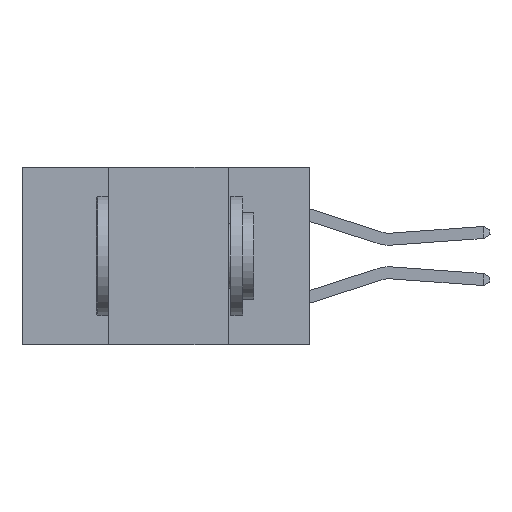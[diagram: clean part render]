
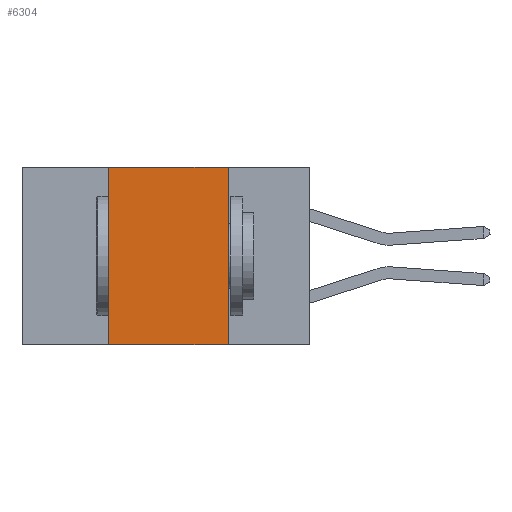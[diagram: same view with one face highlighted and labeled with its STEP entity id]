
A CAD part, left-side view. The second image highlights one B-rep face of the part: STEP entity #6304.
In plain terms, the highlighted planar face has unit normal (-1, 0, 0).
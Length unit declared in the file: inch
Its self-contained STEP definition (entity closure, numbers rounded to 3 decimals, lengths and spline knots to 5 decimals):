
#212 = DIRECTION ( 'NONE',  ( 0., 0., 1. ) ) ;
#338 = ORIENTED_EDGE ( 'NONE', *, *, #6580, .F. ) ;
#1374 = VERTEX_POINT ( 'NONE', #10463 ) ;
#1712 = LINE ( 'NONE', #11741, #5509 ) ;
#1825 = VECTOR ( 'NONE', #12276, 39.37008 ) ;
#3275 = VECTOR ( 'NONE', #7470, 39.37008 ) ;
#4083 = EDGE_CURVE ( 'NONE', #11158, #1374, #1712, .T. ) ;
#4914 = EDGE_CURVE ( 'NONE', #11158, #8663, #6254, .T. ) ;
#5231 = CARTESIAN_POINT ( 'NONE',  ( 0., 0.17, 0. ) ) ;
#5509 = VECTOR ( 'NONE', #11849, 39.37008 ) ;
#5826 = ORIENTED_EDGE ( 'NONE', *, *, #7410, .F. ) ;
#6081 = VERTEX_POINT ( 'NONE', #5231 ) ;
#6254 = LINE ( 'NONE', #12771, #9502 ) ;
#6304 = ADVANCED_FACE ( 'NONE', ( #10438 ), #14697, .F. ) ;
#6580 = EDGE_CURVE ( 'NONE', #8663, #6081, #13028, .T. ) ;
#7289 = CARTESIAN_POINT ( 'NONE',  ( 0., 0.6, 0. ) ) ;
#7410 = EDGE_CURVE ( 'NONE', #6081, #1374, #11324, .T. ) ;
#7470 = DIRECTION ( 'NONE',  ( 0., -1., 0. ) ) ;
#8663 = VERTEX_POINT ( 'NONE', #10891 ) ;
#9502 = VECTOR ( 'NONE', #212, 39.37008 ) ;
#10200 = ORIENTED_EDGE ( 'NONE', *, *, #4914, .F. ) ;
#10438 = FACE_OUTER_BOUND ( 'NONE', #11089, .T. ) ;
#10463 = CARTESIAN_POINT ( 'NONE',  ( 0., 0.17, -0.37 ) ) ;
#10891 = CARTESIAN_POINT ( 'NONE',  ( 0., 0.42, 0. ) ) ;
#11089 = EDGE_LOOP ( 'NONE', ( #5826, #338, #10200, #13727 ) ) ;
#11158 = VERTEX_POINT ( 'NONE', #13565 ) ;
#11324 = LINE ( 'NONE', #12110, #1825 ) ;
#11741 = CARTESIAN_POINT ( 'NONE',  ( 0., 0.6, -0.37 ) ) ;
#11849 = DIRECTION ( 'NONE',  ( 0., -1., 0. ) ) ;
#11993 = AXIS2_PLACEMENT_3D ( 'NONE', #14790, #14634, #14435 ) ;
#12110 = CARTESIAN_POINT ( 'NONE',  ( 0., 0.17, -0.37 ) ) ;
#12276 = DIRECTION ( 'NONE',  ( 0., 0., -1. ) ) ;
#12771 = CARTESIAN_POINT ( 'NONE',  ( 0., 0.42, -0.37 ) ) ;
#13028 = LINE ( 'NONE', #7289, #3275 ) ;
#13565 = CARTESIAN_POINT ( 'NONE',  ( 0., 0.42, -0.37 ) ) ;
#13727 = ORIENTED_EDGE ( 'NONE', *, *, #4083, .T. ) ;
#14435 = DIRECTION ( 'NONE',  ( 0., 0., -1. ) ) ;
#14634 = DIRECTION ( 'NONE',  ( 1., 0., 0. ) ) ;
#14697 = PLANE ( 'NONE',  #11993 ) ;
#14790 = CARTESIAN_POINT ( 'NONE',  ( 0., 0.6, 0. ) ) ;
